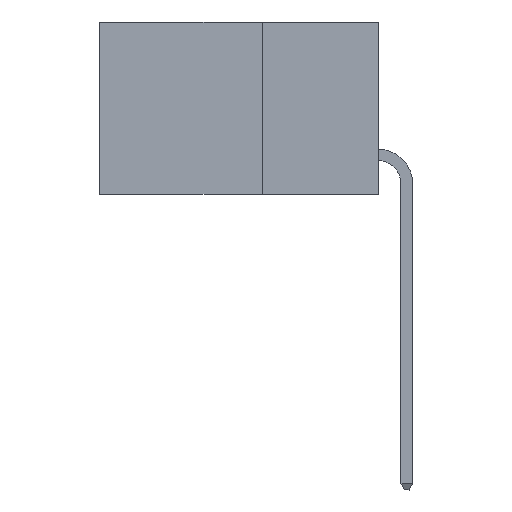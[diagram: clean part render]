
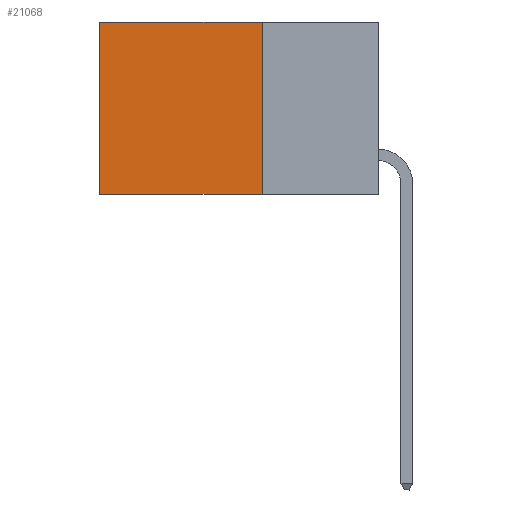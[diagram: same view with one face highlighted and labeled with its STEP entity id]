
A CAD part, left-side view. The second image highlights one B-rep face of the part: STEP entity #21068.
In plain terms, the highlighted planar face has unit normal (-1, 0, 0).
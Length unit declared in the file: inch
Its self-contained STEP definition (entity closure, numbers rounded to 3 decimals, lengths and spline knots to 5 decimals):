
#721 = DIRECTION ( 'NONE',  ( 0., 0., -1. ) ) ;
#2653 = DIRECTION ( 'NONE',  ( 0., 0., -1. ) ) ;
#3580 = EDGE_CURVE ( 'NONE', #13022, #13523, #10523, .T. ) ;
#4624 = VECTOR ( 'NONE', #17025, 39.37008 ) ;
#4988 = FACE_OUTER_BOUND ( 'NONE', #15161, .T. ) ;
#6185 = CARTESIAN_POINT ( 'NONE',  ( 0.298, 0.25, -0.37 ) ) ;
#7428 = EDGE_CURVE ( 'NONE', #24317, #10689, #16395, .T. ) ;
#8254 = CARTESIAN_POINT ( 'NONE',  ( 0.298, 0.25, 0. ) ) ;
#8468 = VECTOR ( 'NONE', #2653, 39.37008 ) ;
#10264 = CARTESIAN_POINT ( 'NONE',  ( 0.298, 0.25, 0. ) ) ;
#10379 = LINE ( 'NONE', #17371, #15429 ) ;
#10436 = DIRECTION ( 'NONE',  ( 0., 1., 0. ) ) ;
#10523 = LINE ( 'NONE', #23463, #4624 ) ;
#10689 = VERTEX_POINT ( 'NONE', #22682 ) ;
#11640 = ORIENTED_EDGE ( 'NONE', *, *, #28033, .F. ) ;
#11709 = PLANE ( 'NONE',  #18596 ) ;
#13022 = VERTEX_POINT ( 'NONE', #6185 ) ;
#13523 = VERTEX_POINT ( 'NONE', #16439 ) ;
#13892 = DIRECTION ( 'NONE',  ( 1., 0., 0. ) ) ;
#13957 = EDGE_CURVE ( 'NONE', #10689, #13523, #25006, .T. ) ;
#15161 = EDGE_LOOP ( 'NONE', ( #17751, #19087, #11640, #21963 ) ) ;
#15429 = VECTOR ( 'NONE', #28153, 39.37008 ) ;
#15759 = CARTESIAN_POINT ( 'NONE',  ( 0.298, 0.6, 0. ) ) ;
#16395 = LINE ( 'NONE', #8254, #27208 ) ;
#16439 = CARTESIAN_POINT ( 'NONE',  ( 0.298, 0.6, -0.37 ) ) ;
#17025 = DIRECTION ( 'NONE',  ( 0., 1., 0. ) ) ;
#17371 = CARTESIAN_POINT ( 'NONE',  ( 0.298, 0.25, 0. ) ) ;
#17751 = ORIENTED_EDGE ( 'NONE', *, *, #13957, .T. ) ;
#18596 = AXIS2_PLACEMENT_3D ( 'NONE', #26820, #13892, #721 ) ;
#19087 = ORIENTED_EDGE ( 'NONE', *, *, #3580, .F. ) ;
#21068 = ADVANCED_FACE ( 'NONE', ( #4988 ), #11709, .F. ) ;
#21963 = ORIENTED_EDGE ( 'NONE', *, *, #7428, .T. ) ;
#22682 = CARTESIAN_POINT ( 'NONE',  ( 0.298, 0.6, 0. ) ) ;
#23463 = CARTESIAN_POINT ( 'NONE',  ( 0.298, 0.25, -0.37 ) ) ;
#24317 = VERTEX_POINT ( 'NONE', #10264 ) ;
#25006 = LINE ( 'NONE', #15759, #8468 ) ;
#26820 = CARTESIAN_POINT ( 'NONE',  ( 0.298, 0.25, 0. ) ) ;
#27208 = VECTOR ( 'NONE', #10436, 39.37008 ) ;
#28033 = EDGE_CURVE ( 'NONE', #24317, #13022, #10379, .T. ) ;
#28153 = DIRECTION ( 'NONE',  ( 0., 0., -1. ) ) ;
